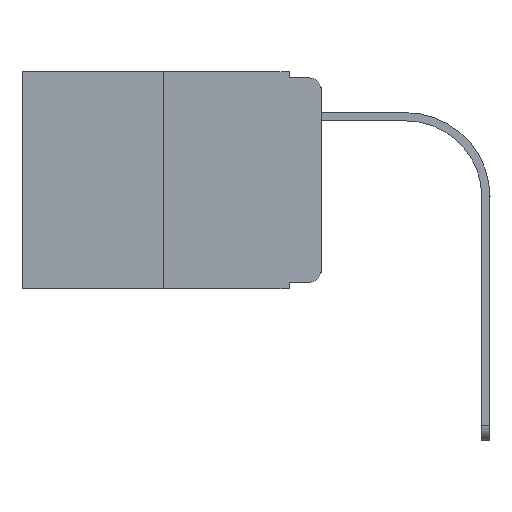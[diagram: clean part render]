
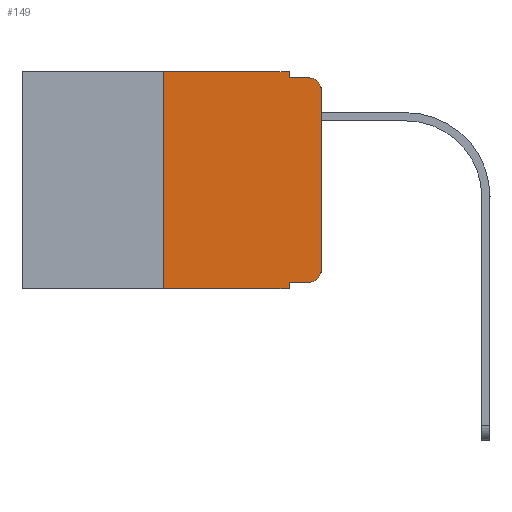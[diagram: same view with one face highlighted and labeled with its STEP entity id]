
A CAD part, left-side view. The second image highlights one B-rep face of the part: STEP entity #149.
In plain terms, the highlighted planar face has unit normal (-1, 0, 0).
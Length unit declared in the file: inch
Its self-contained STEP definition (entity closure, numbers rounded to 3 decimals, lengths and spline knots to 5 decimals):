
#149 = ADVANCED_FACE ( 'NONE', ( #7199 ), #12189, .F. ) ;
#404 = DIRECTION ( 'NONE',  ( 0., 0., -1. ) ) ;
#585 = VECTOR ( 'NONE', #404, 39.37008 ) ;
#806 = CARTESIAN_POINT ( 'NONE',  ( 0., 0.02, -0.01 ) ) ;
#1668 = VECTOR ( 'NONE', #10772, 39.37008 ) ;
#1786 = EDGE_CURVE ( 'NONE', #11508, #4535, #4492, .T. ) ;
#2201 = EDGE_CURVE ( 'NONE', #14193, #10183, #6656, .T. ) ;
#2279 = CARTESIAN_POINT ( 'NONE',  ( 0., 0.02, -0.03 ) ) ;
#2598 = EDGE_LOOP ( 'NONE', ( #13213, #12298, #3416, #14735, #14896, #9733, #16712, #11896, #9671, #7234 ) ) ;
#2757 = CARTESIAN_POINT ( 'NONE',  ( 0., 0.051, -0.343 ) ) ;
#3322 = CARTESIAN_POINT ( 'NONE',  ( 0., 0., -0.03 ) ) ;
#3348 = EDGE_CURVE ( 'NONE', #6297, #4049, #4888, .T. ) ;
#3380 = CARTESIAN_POINT ( 'NONE',  ( 0., 0., 0. ) ) ;
#3416 = ORIENTED_EDGE ( 'NONE', *, *, #6531, .F. ) ;
#4049 = VERTEX_POINT ( 'NONE', #806 ) ;
#4294 = CARTESIAN_POINT ( 'NONE',  ( 0., 0.051, 0. ) ) ;
#4492 = CIRCLE ( 'NONE', #5847, 0.02 ) ;
#4521 = EDGE_CURVE ( 'NONE', #14193, #11947, #16356, .T. ) ;
#4535 = VERTEX_POINT ( 'NONE', #16525 ) ;
#4590 = LINE ( 'NONE', #14927, #1668 ) ;
#4679 = CARTESIAN_POINT ( 'NONE',  ( 0., 0.25, 0. ) ) ;
#4829 = VECTOR ( 'NONE', #6791, 39.37008 ) ;
#4888 = CIRCLE ( 'NONE', #13005, 0.02 ) ;
#5178 = DIRECTION ( 'NONE',  ( 0., 0., -1. ) ) ;
#5227 = CARTESIAN_POINT ( 'NONE',  ( 0., 0.473, -0.343 ) ) ;
#5597 = LINE ( 'NONE', #9172, #8303 ) ;
#5690 = CARTESIAN_POINT ( 'NONE',  ( 0., 0.473, 0. ) ) ;
#5847 = AXIS2_PLACEMENT_3D ( 'NONE', #14157, #7895, #5178 ) ;
#6297 = VERTEX_POINT ( 'NONE', #3322 ) ;
#6531 = EDGE_CURVE ( 'NONE', #10947, #4049, #5597, .T. ) ;
#6656 = LINE ( 'NONE', #5227, #16676 ) ;
#6754 = EDGE_CURVE ( 'NONE', #4535, #6297, #14993, .T. ) ;
#6791 = DIRECTION ( 'NONE',  ( 0., -1., 0. ) ) ;
#6839 = LINE ( 'NONE', #4294, #585 ) ;
#7199 = FACE_OUTER_BOUND ( 'NONE', #2598, .T. ) ;
#7234 = ORIENTED_EDGE ( 'NONE', *, *, #1786, .T. ) ;
#7390 = DIRECTION ( 'NONE',  ( 0., 0., 1. ) ) ;
#7756 = CARTESIAN_POINT ( 'NONE',  ( 0., 0.051, -0.333 ) ) ;
#7775 = CARTESIAN_POINT ( 'NONE',  ( 0., 0.051, 0. ) ) ;
#7895 = DIRECTION ( 'NONE',  ( -1., 0., 0. ) ) ;
#8085 = CARTESIAN_POINT ( 'NONE',  ( 0., 0.25, 0. ) ) ;
#8303 = VECTOR ( 'NONE', #15921, 39.37008 ) ;
#8399 = DIRECTION ( 'NONE',  ( 0., 0., -1. ) ) ;
#8505 = DIRECTION ( 'NONE',  ( 0., 0., -1. ) ) ;
#8949 = VECTOR ( 'NONE', #15189, 39.37008 ) ;
#9172 = CARTESIAN_POINT ( 'NONE',  ( 0., 0.051, -0.01 ) ) ;
#9506 = DIRECTION ( 'NONE',  ( 1., 0., 0. ) ) ;
#9671 = ORIENTED_EDGE ( 'NONE', *, *, #14229, .T. ) ;
#9733 = ORIENTED_EDGE ( 'NONE', *, *, #4521, .F. ) ;
#10183 = VERTEX_POINT ( 'NONE', #2757 ) ;
#10598 = EDGE_CURVE ( 'NONE', #11947, #12639, #10769, .T. ) ;
#10769 = LINE ( 'NONE', #5690, #4829 ) ;
#10772 = DIRECTION ( 'NONE',  ( 0., 0., -1. ) ) ;
#10947 = VERTEX_POINT ( 'NONE', #12699 ) ;
#11180 = CARTESIAN_POINT ( 'NONE',  ( 0., 0.473, 0. ) ) ;
#11508 = VERTEX_POINT ( 'NONE', #15640 ) ;
#11896 = ORIENTED_EDGE ( 'NONE', *, *, #15812, .F. ) ;
#11947 = VERTEX_POINT ( 'NONE', #8085 ) ;
#12189 = PLANE ( 'NONE',  #15950 ) ;
#12298 = ORIENTED_EDGE ( 'NONE', *, *, #3348, .T. ) ;
#12634 = CARTESIAN_POINT ( 'NONE',  ( 0., 0.25, -0.343 ) ) ;
#12639 = VERTEX_POINT ( 'NONE', #7775 ) ;
#12699 = CARTESIAN_POINT ( 'NONE',  ( 0., 0.051, -0.01 ) ) ;
#13005 = AXIS2_PLACEMENT_3D ( 'NONE', #2279, #13818, #8505 ) ;
#13044 = VERTEX_POINT ( 'NONE', #7756 ) ;
#13213 = ORIENTED_EDGE ( 'NONE', *, *, #6754, .T. ) ;
#13273 = DIRECTION ( 'NONE',  ( 0., -1., 0. ) ) ;
#13716 = DIRECTION ( 'NONE',  ( 0., 0., 1. ) ) ;
#13818 = DIRECTION ( 'NONE',  ( -1., 0., 0. ) ) ;
#13992 = LINE ( 'NONE', #16449, #8949 ) ;
#14157 = CARTESIAN_POINT ( 'NONE',  ( 0., 0.02, -0.313 ) ) ;
#14193 = VERTEX_POINT ( 'NONE', #12634 ) ;
#14229 = EDGE_CURVE ( 'NONE', #13044, #11508, #13992, .T. ) ;
#14308 = VECTOR ( 'NONE', #7390, 39.37008 ) ;
#14735 = ORIENTED_EDGE ( 'NONE', *, *, #15254, .F. ) ;
#14896 = ORIENTED_EDGE ( 'NONE', *, *, #10598, .F. ) ;
#14927 = CARTESIAN_POINT ( 'NONE',  ( 0., 0.051, 0. ) ) ;
#14993 = LINE ( 'NONE', #3380, #16411 ) ;
#15189 = DIRECTION ( 'NONE',  ( 0., -1., 0. ) ) ;
#15254 = EDGE_CURVE ( 'NONE', #12639, #10947, #6839, .T. ) ;
#15640 = CARTESIAN_POINT ( 'NONE',  ( 0., 0.02, -0.333 ) ) ;
#15812 = EDGE_CURVE ( 'NONE', #13044, #10183, #4590, .T. ) ;
#15921 = DIRECTION ( 'NONE',  ( 0., -1., 0. ) ) ;
#15950 = AXIS2_PLACEMENT_3D ( 'NONE', #11180, #9506, #8399 ) ;
#16356 = LINE ( 'NONE', #4679, #14308 ) ;
#16411 = VECTOR ( 'NONE', #13716, 39.37008 ) ;
#16449 = CARTESIAN_POINT ( 'NONE',  ( 0., 0.051, -0.333 ) ) ;
#16525 = CARTESIAN_POINT ( 'NONE',  ( 0., 0., -0.313 ) ) ;
#16676 = VECTOR ( 'NONE', #13273, 39.37008 ) ;
#16712 = ORIENTED_EDGE ( 'NONE', *, *, #2201, .T. ) ;
